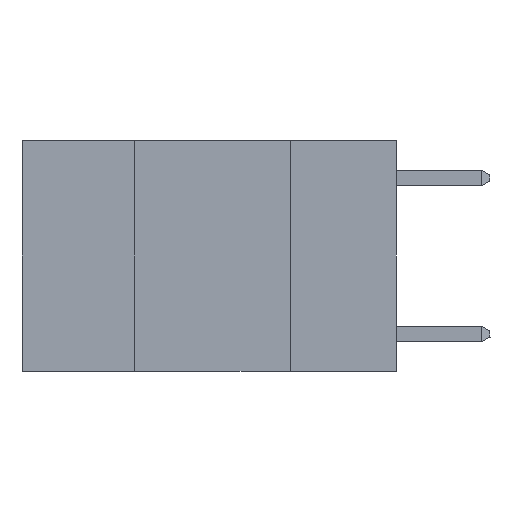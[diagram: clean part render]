
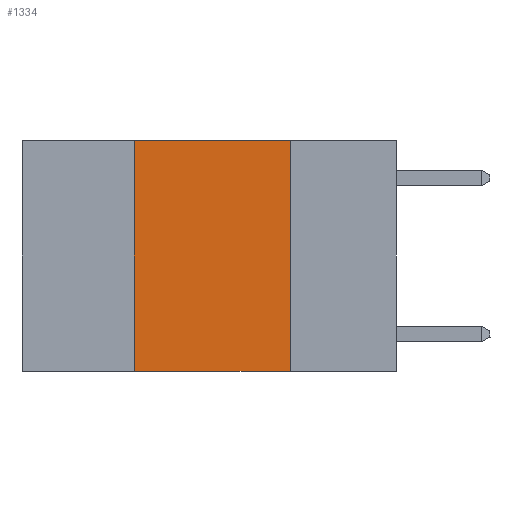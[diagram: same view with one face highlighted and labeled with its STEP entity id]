
A CAD part, left-side view. The second image highlights one B-rep face of the part: STEP entity #1334.
In plain terms, the highlighted planar face has unit normal (-1, 0, 0).
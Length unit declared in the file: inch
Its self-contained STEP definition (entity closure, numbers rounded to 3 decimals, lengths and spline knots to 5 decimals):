
#394 = DIRECTION ( 'NONE',  ( 1., 0., 0. ) ) ;
#423 = VECTOR ( 'NONE', #3159, 39.37008 ) ;
#1037 = CARTESIAN_POINT ( 'NONE',  ( 0., 0.17, 0. ) ) ;
#1334 = ADVANCED_FACE ( 'NONE', ( #5878 ), #20070, .F. ) ;
#1521 = VERTEX_POINT ( 'NONE', #1037 ) ;
#1566 = VERTEX_POINT ( 'NONE', #10391 ) ;
#2194 = CARTESIAN_POINT ( 'NONE',  ( 0., 0.6, 0. ) ) ;
#2845 = CARTESIAN_POINT ( 'NONE',  ( 0., 0.42, -0.37 ) ) ;
#3159 = DIRECTION ( 'NONE',  ( 0., -1., 0. ) ) ;
#3265 = VECTOR ( 'NONE', #18814, 39.37008 ) ;
#3743 = VERTEX_POINT ( 'NONE', #2845 ) ;
#5459 = AXIS2_PLACEMENT_3D ( 'NONE', #2194, #394, #13141 ) ;
#5726 = VERTEX_POINT ( 'NONE', #12050 ) ;
#5878 = FACE_OUTER_BOUND ( 'NONE', #14155, .T. ) ;
#6825 = LINE ( 'NONE', #22689, #11009 ) ;
#8818 = VECTOR ( 'NONE', #13432, 39.37008 ) ;
#10391 = CARTESIAN_POINT ( 'NONE',  ( 0., 0.42, 0. ) ) ;
#11009 = VECTOR ( 'NONE', #14249, 39.37008 ) ;
#11755 = CARTESIAN_POINT ( 'NONE',  ( 0., 0.17, 0. ) ) ;
#12050 = CARTESIAN_POINT ( 'NONE',  ( 0., 0.17, -0.37 ) ) ;
#13141 = DIRECTION ( 'NONE',  ( 0., 0., -1. ) ) ;
#13432 = DIRECTION ( 'NONE',  ( 0., -1., 0. ) ) ;
#13513 = LINE ( 'NONE', #16954, #8818 ) ;
#13957 = CARTESIAN_POINT ( 'NONE',  ( 0., 0.6, 0. ) ) ;
#14155 = EDGE_LOOP ( 'NONE', ( #17830, #18160, #18515, #17781 ) ) ;
#14249 = DIRECTION ( 'NONE',  ( 0., 0., 1. ) ) ;
#15718 = EDGE_CURVE ( 'NONE', #1566, #1521, #18482, .T. ) ;
#16781 = EDGE_CURVE ( 'NONE', #3743, #5726, #13513, .T. ) ;
#16954 = CARTESIAN_POINT ( 'NONE',  ( 0., 0.6, -0.37 ) ) ;
#17578 = LINE ( 'NONE', #11755, #3265 ) ;
#17781 = ORIENTED_EDGE ( 'NONE', *, *, #16781, .T. ) ;
#17830 = ORIENTED_EDGE ( 'NONE', *, *, #19058, .F. ) ;
#17920 = EDGE_CURVE ( 'NONE', #3743, #1566, #6825, .T. ) ;
#18160 = ORIENTED_EDGE ( 'NONE', *, *, #15718, .F. ) ;
#18482 = LINE ( 'NONE', #13957, #423 ) ;
#18515 = ORIENTED_EDGE ( 'NONE', *, *, #17920, .F. ) ;
#18814 = DIRECTION ( 'NONE',  ( 0., 0., -1. ) ) ;
#19058 = EDGE_CURVE ( 'NONE', #1521, #5726, #17578, .T. ) ;
#20070 = PLANE ( 'NONE',  #5459 ) ;
#22689 = CARTESIAN_POINT ( 'NONE',  ( 0., 0.42, 0. ) ) ;
